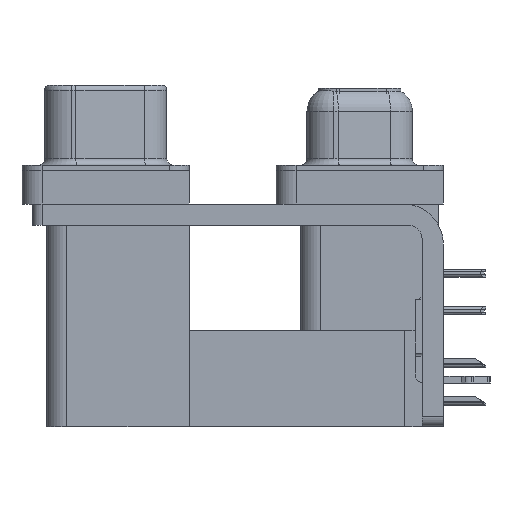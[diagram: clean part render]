
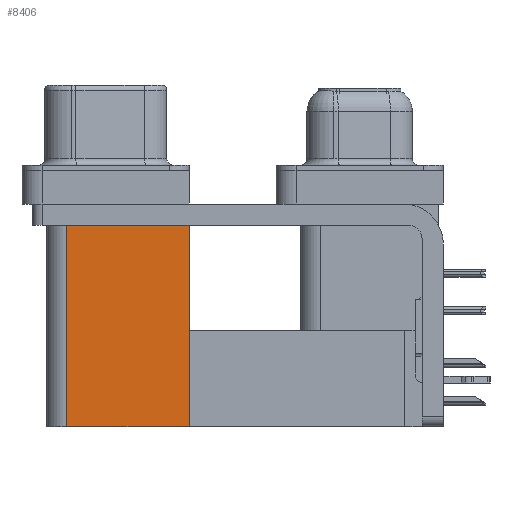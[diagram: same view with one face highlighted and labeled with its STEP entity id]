
A CAD part, left-side view. The second image highlights one B-rep face of the part: STEP entity #8406.
In plain terms, the highlighted planar face has unit normal (-1, 0, 0).
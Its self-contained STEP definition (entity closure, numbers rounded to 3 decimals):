
#232 = ORIENTED_EDGE ( 'NONE', *, *, #4786, .F. ) ;
#1010 = EDGE_LOOP ( 'NONE', ( #8622, #232, #2236, #48158 ) ) ;
#2236 = ORIENTED_EDGE ( 'NONE', *, *, #31272, .F. ) ;
#2371 = LINE ( 'NONE', #48026, #29918 ) ;
#4710 = FACE_OUTER_BOUND ( 'NONE', #1010, .T. ) ;
#4786 = EDGE_CURVE ( 'NONE', #53630, #18261, #9829, .T. ) ;
#5158 = CARTESIAN_POINT ( 'NONE',  ( 3.7, 21.975, -19.2 ) ) ;
#6094 = CARTESIAN_POINT ( 'NONE',  ( 3.7, 12.775, -2.5 ) ) ;
#7749 = CARTESIAN_POINT ( 'NONE',  ( 3.7, 21.975, -2.5 ) ) ;
#8406 = ADVANCED_FACE ( 'NONE', ( #4710 ), #21503, .F. ) ;
#8622 = ORIENTED_EDGE ( 'NONE', *, *, #30366, .T. ) ;
#9829 = LINE ( 'NONE', #5158, #24958 ) ;
#14730 = CARTESIAN_POINT ( 'NONE',  ( 3.7, 12.775, -19.2 ) ) ;
#16308 = LINE ( 'NONE', #24272, #21053 ) ;
#17294 = DIRECTION ( 'NONE',  ( 0., 0., 1. ) ) ;
#18261 = VERTEX_POINT ( 'NONE', #7749 ) ;
#20949 = DIRECTION ( 'NONE',  ( 1., 0., 0. ) ) ;
#21053 = VECTOR ( 'NONE', #49553, 1000. ) ;
#21222 = CARTESIAN_POINT ( 'NONE',  ( 3.7, 12.775, -19.2 ) ) ;
#21503 = PLANE ( 'NONE',  #40503 ) ;
#24272 = CARTESIAN_POINT ( 'NONE',  ( 3.7, 12.775, -2.5 ) ) ;
#24958 = VECTOR ( 'NONE', #17294, 1000. ) ;
#29918 = VECTOR ( 'NONE', #52682, 1000. ) ;
#30366 = EDGE_CURVE ( 'NONE', #30657, #18261, #16308, .T. ) ;
#30657 = VERTEX_POINT ( 'NONE', #6094 ) ;
#30697 = CARTESIAN_POINT ( 'NONE',  ( 3.7, 21.975, -19.2 ) ) ;
#31272 = EDGE_CURVE ( 'NONE', #32886, #53630, #2371, .T. ) ;
#32024 = EDGE_CURVE ( 'NONE', #32886, #30657, #51764, .T. ) ;
#32886 = VERTEX_POINT ( 'NONE', #14730 ) ;
#37703 = DIRECTION ( 'NONE',  ( 0., 1., 0. ) ) ;
#40503 = AXIS2_PLACEMENT_3D ( 'NONE', #21222, #20949, #37703 ) ;
#43161 = VECTOR ( 'NONE', #47094, 1000. ) ;
#47094 = DIRECTION ( 'NONE',  ( 0., 0., 1. ) ) ;
#48026 = CARTESIAN_POINT ( 'NONE',  ( 3.7, 12.775, -19.2 ) ) ;
#48158 = ORIENTED_EDGE ( 'NONE', *, *, #32024, .T. ) ;
#49553 = DIRECTION ( 'NONE',  ( 0., 1., 0. ) ) ;
#51764 = LINE ( 'NONE', #52026, #43161 ) ;
#52026 = CARTESIAN_POINT ( 'NONE',  ( 3.7, 12.775, -19.2 ) ) ;
#52682 = DIRECTION ( 'NONE',  ( 0., 1., 0. ) ) ;
#53630 = VERTEX_POINT ( 'NONE', #30697 ) ;
